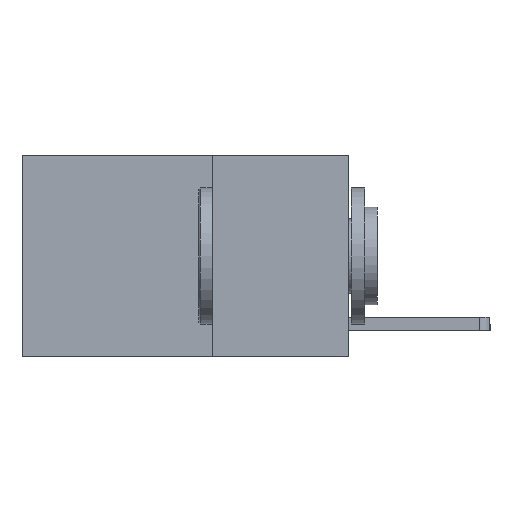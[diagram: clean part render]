
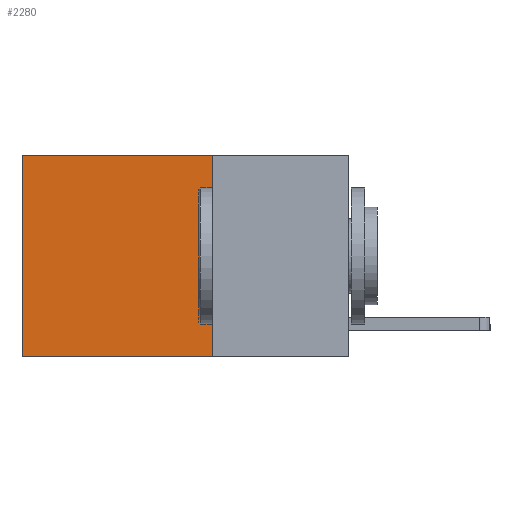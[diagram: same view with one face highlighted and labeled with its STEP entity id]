
A CAD part, left-side view. The second image highlights one B-rep face of the part: STEP entity #2280.
In plain terms, the highlighted planar face has unit normal (-1, 0, 0).
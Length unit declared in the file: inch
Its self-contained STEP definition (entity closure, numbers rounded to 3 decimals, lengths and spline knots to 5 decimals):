
#4 = VECTOR ( 'NONE', #7966, 39.37008 ) ;
#61 = EDGE_CURVE ( 'NONE', #3024, #8844, #8813, .T. ) ;
#79 = EDGE_LOOP ( 'NONE', ( #4209, #2810, #7242, #6200 ) ) ;
#653 = CARTESIAN_POINT ( 'NONE',  ( 0.2625, 0.25, -0.37 ) ) ;
#703 = EDGE_CURVE ( 'NONE', #3024, #2046, #10725, .T. ) ;
#1138 = DIRECTION ( 'NONE',  ( 0., 0., -1. ) ) ;
#1163 = CARTESIAN_POINT ( 'NONE',  ( 0.2625, 0.25, 0. ) ) ;
#1599 = CARTESIAN_POINT ( 'NONE',  ( 0.2625, 0.6, 0. ) ) ;
#1692 = LINE ( 'NONE', #10089, #6662 ) ;
#2027 = DIRECTION ( 'NONE',  ( 1., 0., 0. ) ) ;
#2046 = VERTEX_POINT ( 'NONE', #653 ) ;
#2280 = ADVANCED_FACE ( 'NONE', ( #6135 ), #9518, .F. ) ;
#2525 = CARTESIAN_POINT ( 'NONE',  ( 0.2625, 0.25, 0. ) ) ;
#2569 = EDGE_CURVE ( 'NONE', #2046, #9712, #1692, .T. ) ;
#2810 = ORIENTED_EDGE ( 'NONE', *, *, #2569, .F. ) ;
#3024 = VERTEX_POINT ( 'NONE', #2525 ) ;
#3096 = VECTOR ( 'NONE', #7722, 39.37008 ) ;
#3233 = AXIS2_PLACEMENT_3D ( 'NONE', #7035, #2027, #1138 ) ;
#4082 = VECTOR ( 'NONE', #8186, 39.37008 ) ;
#4209 = ORIENTED_EDGE ( 'NONE', *, *, #6598, .T. ) ;
#5535 = CARTESIAN_POINT ( 'NONE',  ( 0.2625, 0.25, 0. ) ) ;
#5813 = CARTESIAN_POINT ( 'NONE',  ( 0.2625, 0.6, 0. ) ) ;
#6135 = FACE_OUTER_BOUND ( 'NONE', #79, .T. ) ;
#6200 = ORIENTED_EDGE ( 'NONE', *, *, #61, .T. ) ;
#6521 = CARTESIAN_POINT ( 'NONE',  ( 0.2625, 0.6, -0.37 ) ) ;
#6598 = EDGE_CURVE ( 'NONE', #8844, #9712, #7618, .T. ) ;
#6662 = VECTOR ( 'NONE', #9337, 39.37008 ) ;
#7035 = CARTESIAN_POINT ( 'NONE',  ( 0.2625, 0.25, 0. ) ) ;
#7242 = ORIENTED_EDGE ( 'NONE', *, *, #703, .F. ) ;
#7618 = LINE ( 'NONE', #1599, #3096 ) ;
#7722 = DIRECTION ( 'NONE',  ( 0., 0., -1. ) ) ;
#7966 = DIRECTION ( 'NONE',  ( 0., 1., 0. ) ) ;
#8186 = DIRECTION ( 'NONE',  ( 0., 0., -1. ) ) ;
#8813 = LINE ( 'NONE', #1163, #4 ) ;
#8844 = VERTEX_POINT ( 'NONE', #5813 ) ;
#9337 = DIRECTION ( 'NONE',  ( 0., 1., 0. ) ) ;
#9518 = PLANE ( 'NONE',  #3233 ) ;
#9712 = VERTEX_POINT ( 'NONE', #6521 ) ;
#10089 = CARTESIAN_POINT ( 'NONE',  ( 0.2625, 0.25, -0.37 ) ) ;
#10725 = LINE ( 'NONE', #5535, #4082 ) ;
